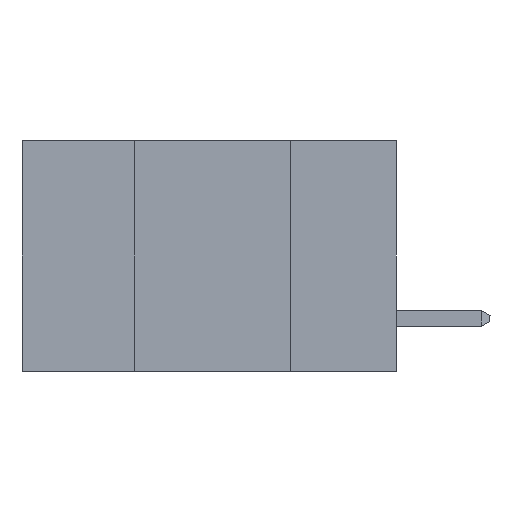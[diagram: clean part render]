
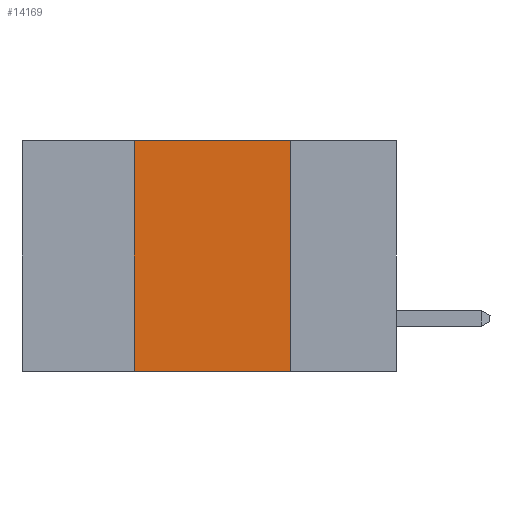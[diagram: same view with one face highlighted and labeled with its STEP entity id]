
A CAD part, left-side view. The second image highlights one B-rep face of the part: STEP entity #14169.
In plain terms, the highlighted planar face has unit normal (-1, 0, 0).
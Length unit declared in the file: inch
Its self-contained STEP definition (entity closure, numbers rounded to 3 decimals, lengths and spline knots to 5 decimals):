
#837 = VERTEX_POINT ( 'NONE', #6375 ) ;
#998 = EDGE_CURVE ( 'NONE', #837, #11977, #9236, .T. ) ;
#1232 = DIRECTION ( 'NONE',  ( 0., 0., -1. ) ) ;
#2592 = CARTESIAN_POINT ( 'NONE',  ( 0., 0.6, -0.37 ) ) ;
#2707 = CARTESIAN_POINT ( 'NONE',  ( 0., 0.17, -0.37 ) ) ;
#2865 = EDGE_LOOP ( 'NONE', ( #6485, #15710, #5990, #8304 ) ) ;
#4802 = VECTOR ( 'NONE', #11294, 39.37008 ) ;
#4815 = LINE ( 'NONE', #15333, #11063 ) ;
#5990 = ORIENTED_EDGE ( 'NONE', *, *, #15355, .F. ) ;
#6375 = CARTESIAN_POINT ( 'NONE',  ( 0., 0.42, -0.37 ) ) ;
#6485 = ORIENTED_EDGE ( 'NONE', *, *, #7964, .F. ) ;
#6847 = FACE_OUTER_BOUND ( 'NONE', #2865, .T. ) ;
#7193 = LINE ( 'NONE', #11020, #10475 ) ;
#7285 = CARTESIAN_POINT ( 'NONE',  ( 0., 0.17, 0. ) ) ;
#7520 = CARTESIAN_POINT ( 'NONE',  ( 0., 0.6, 0. ) ) ;
#7964 = EDGE_CURVE ( 'NONE', #14069, #11977, #4815, .T. ) ;
#8304 = ORIENTED_EDGE ( 'NONE', *, *, #998, .T. ) ;
#8559 = LINE ( 'NONE', #10056, #4802 ) ;
#8757 = DIRECTION ( 'NONE',  ( 1., 0., 0. ) ) ;
#9236 = LINE ( 'NONE', #2592, #12071 ) ;
#9421 = DIRECTION ( 'NONE',  ( 0., 0., -1. ) ) ;
#10056 = CARTESIAN_POINT ( 'NONE',  ( 0., 0.6, 0. ) ) ;
#10475 = VECTOR ( 'NONE', #13409, 39.37008 ) ;
#10552 = DIRECTION ( 'NONE',  ( 0., -1., 0. ) ) ;
#11020 = CARTESIAN_POINT ( 'NONE',  ( 0., 0.42, -0.37 ) ) ;
#11063 = VECTOR ( 'NONE', #9421, 39.37008 ) ;
#11294 = DIRECTION ( 'NONE',  ( 0., -1., 0. ) ) ;
#11876 = CARTESIAN_POINT ( 'NONE',  ( 0., 0.42, 0. ) ) ;
#11977 = VERTEX_POINT ( 'NONE', #2707 ) ;
#12071 = VECTOR ( 'NONE', #10552, 39.37008 ) ;
#12561 = AXIS2_PLACEMENT_3D ( 'NONE', #7520, #8757, #1232 ) ;
#13409 = DIRECTION ( 'NONE',  ( 0., 0., 1. ) ) ;
#13491 = PLANE ( 'NONE',  #12561 ) ;
#14069 = VERTEX_POINT ( 'NONE', #7285 ) ;
#14169 = ADVANCED_FACE ( 'NONE', ( #6847 ), #13491, .F. ) ;
#15333 = CARTESIAN_POINT ( 'NONE',  ( 0., 0.17, -0.37 ) ) ;
#15355 = EDGE_CURVE ( 'NONE', #837, #15731, #7193, .T. ) ;
#15471 = EDGE_CURVE ( 'NONE', #15731, #14069, #8559, .T. ) ;
#15710 = ORIENTED_EDGE ( 'NONE', *, *, #15471, .F. ) ;
#15731 = VERTEX_POINT ( 'NONE', #11876 ) ;
